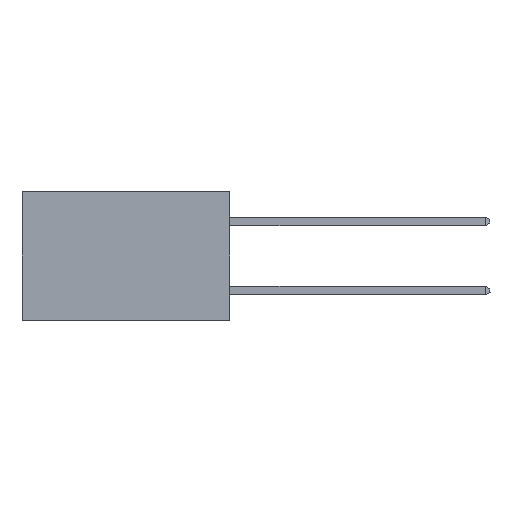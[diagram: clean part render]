
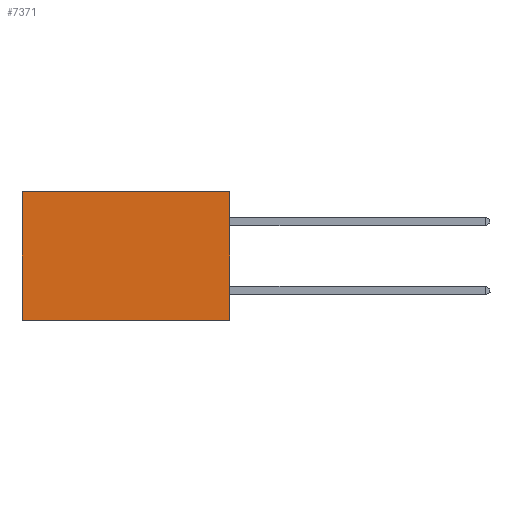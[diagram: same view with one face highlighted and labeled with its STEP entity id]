
A CAD part, left-side view. The second image highlights one B-rep face of the part: STEP entity #7371.
In plain terms, the highlighted planar face has unit normal (-1, 0, 0).
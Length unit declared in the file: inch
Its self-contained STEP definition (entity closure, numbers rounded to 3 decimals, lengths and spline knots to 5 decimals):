
#158 = CARTESIAN_POINT ( 'NONE',  ( 0.298, 0., 0. ) ) ;
#725 = CARTESIAN_POINT ( 'NONE',  ( 0.298, 0.6, 0. ) ) ;
#827 = ORIENTED_EDGE ( 'NONE', *, *, #4128, .F. ) ;
#885 = ORIENTED_EDGE ( 'NONE', *, *, #3575, .F. ) ;
#926 = LINE ( 'NONE', #158, #8532 ) ;
#1618 = PLANE ( 'NONE',  #5948 ) ;
#1662 = DIRECTION ( 'NONE',  ( 1., 0., 0. ) ) ;
#2597 = VERTEX_POINT ( 'NONE', #5524 ) ;
#3366 = VECTOR ( 'NONE', #7743, 39.37008 ) ;
#3387 = VERTEX_POINT ( 'NONE', #12033 ) ;
#3575 = EDGE_CURVE ( 'NONE', #8129, #3387, #3860, .T. ) ;
#3860 = LINE ( 'NONE', #8705, #11000 ) ;
#4123 = DIRECTION ( 'NONE',  ( 0., 1., 0. ) ) ;
#4128 = EDGE_CURVE ( 'NONE', #2597, #8129, #926, .T. ) ;
#4304 = CARTESIAN_POINT ( 'NONE',  ( 0.298, 0., 0. ) ) ;
#4407 = CARTESIAN_POINT ( 'NONE',  ( 0.298, 0., 0. ) ) ;
#5524 = CARTESIAN_POINT ( 'NONE',  ( 0.298, 0., 0. ) ) ;
#5836 = LINE ( 'NONE', #9727, #3366 ) ;
#5948 = AXIS2_PLACEMENT_3D ( 'NONE', #4407, #1662, #9005 ) ;
#7022 = DIRECTION ( 'NONE',  ( 0., 1., 0. ) ) ;
#7331 = CARTESIAN_POINT ( 'NONE',  ( 0.298, 0., -0.37 ) ) ;
#7341 = FACE_OUTER_BOUND ( 'NONE', #10031, .T. ) ;
#7371 = ADVANCED_FACE ( 'NONE', ( #7341 ), #1618, .F. ) ;
#7743 = DIRECTION ( 'NONE',  ( 0., 0., -1. ) ) ;
#8129 = VERTEX_POINT ( 'NONE', #7331 ) ;
#8332 = EDGE_CURVE ( 'NONE', #10427, #3387, #5836, .T. ) ;
#8407 = ORIENTED_EDGE ( 'NONE', *, *, #9693, .T. ) ;
#8532 = VECTOR ( 'NONE', #11277, 39.37008 ) ;
#8705 = CARTESIAN_POINT ( 'NONE',  ( 0.298, 0., -0.37 ) ) ;
#9005 = DIRECTION ( 'NONE',  ( 0., 0., -1. ) ) ;
#9043 = VECTOR ( 'NONE', #7022, 39.37008 ) ;
#9693 = EDGE_CURVE ( 'NONE', #2597, #10427, #10196, .T. ) ;
#9727 = CARTESIAN_POINT ( 'NONE',  ( 0.298, 0.6, 0. ) ) ;
#10031 = EDGE_LOOP ( 'NONE', ( #11299, #885, #827, #8407 ) ) ;
#10196 = LINE ( 'NONE', #4304, #9043 ) ;
#10427 = VERTEX_POINT ( 'NONE', #725 ) ;
#11000 = VECTOR ( 'NONE', #4123, 39.37008 ) ;
#11277 = DIRECTION ( 'NONE',  ( 0., 0., -1. ) ) ;
#11299 = ORIENTED_EDGE ( 'NONE', *, *, #8332, .T. ) ;
#12033 = CARTESIAN_POINT ( 'NONE',  ( 0.298, 0.6, -0.37 ) ) ;
